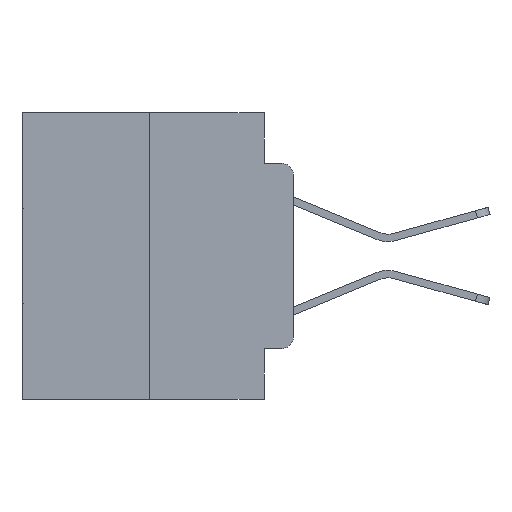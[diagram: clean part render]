
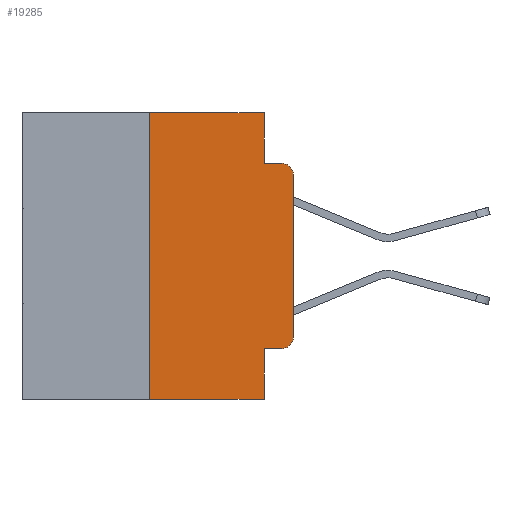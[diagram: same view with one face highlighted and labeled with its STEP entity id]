
A CAD part, left-side view. The second image highlights one B-rep face of the part: STEP entity #19285.
In plain terms, the highlighted planar face has unit normal (-1, 0, 0).
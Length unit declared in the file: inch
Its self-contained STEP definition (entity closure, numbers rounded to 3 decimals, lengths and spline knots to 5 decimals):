
#80 = DIRECTION ( 'NONE',  ( 0., 0., 1. ) ) ;
#591 = EDGE_CURVE ( 'NONE', #22459, #21942, #22483, .T. ) ;
#999 = ORIENTED_EDGE ( 'NONE', *, *, #591, .T. ) ;
#1047 = CARTESIAN_POINT ( 'NONE',  ( 0., 0.051, -0.4115 ) ) ;
#1397 = VECTOR ( 'NONE', #80, 39.37008 ) ;
#1452 = VERTEX_POINT ( 'NONE', #16639 ) ;
#1775 = ORIENTED_EDGE ( 'NONE', *, *, #27264, .T. ) ;
#3223 = ORIENTED_EDGE ( 'NONE', *, *, #27353, .F. ) ;
#3661 = AXIS2_PLACEMENT_3D ( 'NONE', #6692, #8962, #21791 ) ;
#4102 = VECTOR ( 'NONE', #18640, 39.37008 ) ;
#4619 = CARTESIAN_POINT ( 'NONE',  ( 0., 0.473, 0. ) ) ;
#4792 = LINE ( 'NONE', #9699, #7178 ) ;
#4940 = CARTESIAN_POINT ( 'NONE',  ( 0., 0.051, -0.0885 ) ) ;
#5121 = ORIENTED_EDGE ( 'NONE', *, *, #8060, .F. ) ;
#5692 = EDGE_CURVE ( 'NONE', #10553, #26230, #21694, .T. ) ;
#5959 = CARTESIAN_POINT ( 'NONE',  ( 0., 0.02, -0.3915 ) ) ;
#6692 = CARTESIAN_POINT ( 'NONE',  ( 0., 0.02, -0.1085 ) ) ;
#7178 = VECTOR ( 'NONE', #26794, 39.37008 ) ;
#8005 = CIRCLE ( 'NONE', #3661, 0.02 ) ;
#8060 = EDGE_CURVE ( 'NONE', #21321, #21942, #23597, .T. ) ;
#8111 = CARTESIAN_POINT ( 'NONE',  ( 0., 0.051, 0. ) ) ;
#8206 = VECTOR ( 'NONE', #14605, 39.37008 ) ;
#8299 = EDGE_CURVE ( 'NONE', #27287, #16987, #15027, .T. ) ;
#8962 = DIRECTION ( 'NONE',  ( -1., 0., 0. ) ) ;
#9166 = PLANE ( 'NONE',  #15612 ) ;
#9585 = LINE ( 'NONE', #21769, #1397 ) ;
#9699 = CARTESIAN_POINT ( 'NONE',  ( 0., 0.473, 0. ) ) ;
#9778 = CARTESIAN_POINT ( 'NONE',  ( 0., 0.02, -0.0885 ) ) ;
#10072 = VECTOR ( 'NONE', #24520, 39.37008 ) ;
#10553 = VERTEX_POINT ( 'NONE', #4940 ) ;
#10879 = VECTOR ( 'NONE', #24056, 39.37008 ) ;
#11403 = DIRECTION ( 'NONE',  ( 1., 0., 0. ) ) ;
#11994 = VERTEX_POINT ( 'NONE', #27012 ) ;
#12347 = CARTESIAN_POINT ( 'NONE',  ( 0., 0., -0.1085 ) ) ;
#12348 = VECTOR ( 'NONE', #18258, 39.37008 ) ;
#13166 = EDGE_CURVE ( 'NONE', #22459, #11994, #9585, .T. ) ;
#13458 = EDGE_CURVE ( 'NONE', #11994, #23976, #4792, .T. ) ;
#14301 = ORIENTED_EDGE ( 'NONE', *, *, #13166, .F. ) ;
#14444 = ORIENTED_EDGE ( 'NONE', *, *, #5692, .F. ) ;
#14605 = DIRECTION ( 'NONE',  ( 0., 0., -1. ) ) ;
#14884 = FACE_OUTER_BOUND ( 'NONE', #19246, .T. ) ;
#15027 = LINE ( 'NONE', #19193, #20530 ) ;
#15612 = AXIS2_PLACEMENT_3D ( 'NONE', #4619, #11403, #19909 ) ;
#16256 = ORIENTED_EDGE ( 'NONE', *, *, #13458, .F. ) ;
#16639 = CARTESIAN_POINT ( 'NONE',  ( 0., 0.02, -0.4115 ) ) ;
#16987 = VERTEX_POINT ( 'NONE', #12347 ) ;
#17650 = ORIENTED_EDGE ( 'NONE', *, *, #23296, .T. ) ;
#18057 = CIRCLE ( 'NONE', #25932, 0.02 ) ;
#18072 = CARTESIAN_POINT ( 'NONE',  ( 0., 0.051, -0.0885 ) ) ;
#18170 = CARTESIAN_POINT ( 'NONE',  ( 0., 0., -0.3915 ) ) ;
#18258 = DIRECTION ( 'NONE',  ( 0., -1., 0. ) ) ;
#18640 = DIRECTION ( 'NONE',  ( 0., 0., -1. ) ) ;
#18961 = DIRECTION ( 'NONE',  ( -1., 0., 0. ) ) ;
#19193 = CARTESIAN_POINT ( 'NONE',  ( 0., 0., 0. ) ) ;
#19246 = EDGE_LOOP ( 'NONE', ( #27493, #23489, #14444, #3223, #16256, #14301, #999, #5121, #1775, #17650 ) ) ;
#19285 = ADVANCED_FACE ( 'NONE', ( #14884 ), #9166, .F. ) ;
#19909 = DIRECTION ( 'NONE',  ( 0., 0., -1. ) ) ;
#20530 = VECTOR ( 'NONE', #23653, 39.37008 ) ;
#20731 = CARTESIAN_POINT ( 'NONE',  ( 0., 0.051, 0. ) ) ;
#21151 = DIRECTION ( 'NONE',  ( 0., 0., -1. ) ) ;
#21321 = VERTEX_POINT ( 'NONE', #27120 ) ;
#21694 = LINE ( 'NONE', #18072, #10072 ) ;
#21769 = CARTESIAN_POINT ( 'NONE',  ( 0., 0.25, 0. ) ) ;
#21791 = DIRECTION ( 'NONE',  ( 0., 0., -1. ) ) ;
#21797 = CARTESIAN_POINT ( 'NONE',  ( 0., 0.473, -0.5 ) ) ;
#21942 = VERTEX_POINT ( 'NONE', #23265 ) ;
#22459 = VERTEX_POINT ( 'NONE', #24311 ) ;
#22483 = LINE ( 'NONE', #21797, #10879 ) ;
#23265 = CARTESIAN_POINT ( 'NONE',  ( 0., 0.051, -0.5 ) ) ;
#23296 = EDGE_CURVE ( 'NONE', #1452, #27287, #18057, .T. ) ;
#23489 = ORIENTED_EDGE ( 'NONE', *, *, #25146, .T. ) ;
#23597 = LINE ( 'NONE', #20731, #4102 ) ;
#23653 = DIRECTION ( 'NONE',  ( 0., 0., 1. ) ) ;
#23976 = VERTEX_POINT ( 'NONE', #8111 ) ;
#24056 = DIRECTION ( 'NONE',  ( 0., -1., 0. ) ) ;
#24311 = CARTESIAN_POINT ( 'NONE',  ( 0., 0.25, -0.5 ) ) ;
#24520 = DIRECTION ( 'NONE',  ( 0., -1., 0. ) ) ;
#24718 = CARTESIAN_POINT ( 'NONE',  ( 0., 0.051, 0. ) ) ;
#25146 = EDGE_CURVE ( 'NONE', #16987, #26230, #8005, .T. ) ;
#25303 = LINE ( 'NONE', #24718, #8206 ) ;
#25932 = AXIS2_PLACEMENT_3D ( 'NONE', #5959, #18961, #21151 ) ;
#26230 = VERTEX_POINT ( 'NONE', #9778 ) ;
#26794 = DIRECTION ( 'NONE',  ( 0., -1., 0. ) ) ;
#27012 = CARTESIAN_POINT ( 'NONE',  ( 0., 0.25, 0. ) ) ;
#27120 = CARTESIAN_POINT ( 'NONE',  ( 0., 0.051, -0.4115 ) ) ;
#27264 = EDGE_CURVE ( 'NONE', #21321, #1452, #27661, .T. ) ;
#27287 = VERTEX_POINT ( 'NONE', #18170 ) ;
#27353 = EDGE_CURVE ( 'NONE', #23976, #10553, #25303, .T. ) ;
#27493 = ORIENTED_EDGE ( 'NONE', *, *, #8299, .T. ) ;
#27661 = LINE ( 'NONE', #1047, #12348 ) ;
